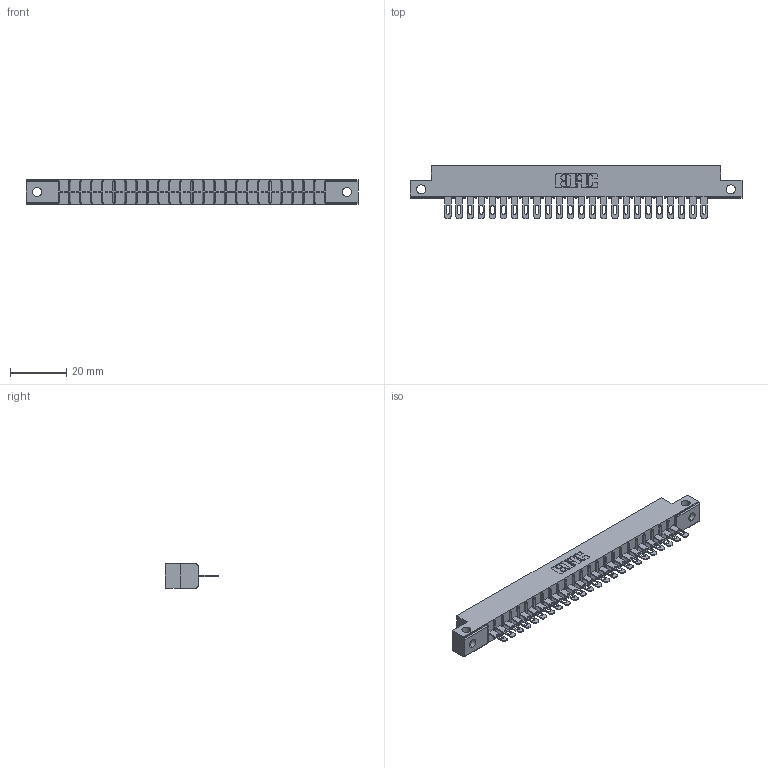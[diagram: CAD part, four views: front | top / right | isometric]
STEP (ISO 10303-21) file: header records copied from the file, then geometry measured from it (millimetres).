
FILE_DESCRIPTION (( 'STEP AP203' ), '1' );
FILE_NAME ('316-024-400-112.STEP', '2020-09-22T21:20:37', ( '' ), ( '' ), 'SwSTEP 2.0', 'SolidWorks 2020', '' );
FILE_SCHEMA (( 'CONFIG_CONTROL_DESIGN' ));
Length unit declared in the file: inch
Products named in the file (3): 316-024-400-112; 306-290-001_100; 306 Part_.128 Dia
Assembly tree (25 placements, depth 2):
  316-024-400-112
    306 Part_.128 Dia
    306-290-001_100  x24
Bounding box: 118.11 x 18.87 x 8.71 mm (x, y, z)
Volume: 8032.3 mm3; surface area: 12256.3 mm2
Topology: 25 solids, 25 shells, 1952 faces, 5512 edges, 3540 vertices
Faces by surface type: plane 1268, cylinder 588, sphere 96
Entity records: 25283 total; most frequent: CARTESIAN_POINT 4291, ORIENTED_EDGE 4208, DIRECTION 4172, EDGE_CURVE 2104, VECTOR 1618, LINE 1618, VERTEX_POINT 1332, AXIS2_PLACEMENT_3D 1277
